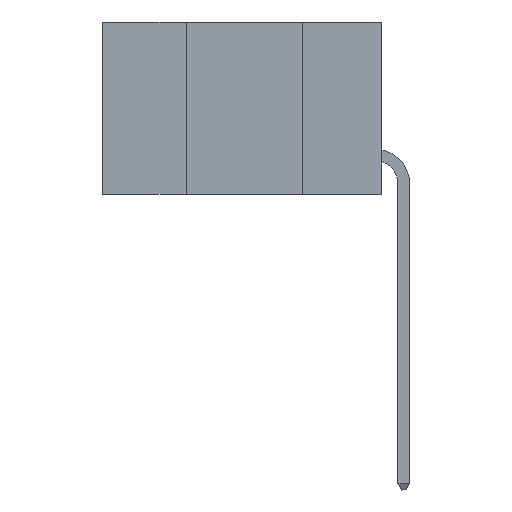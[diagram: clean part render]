
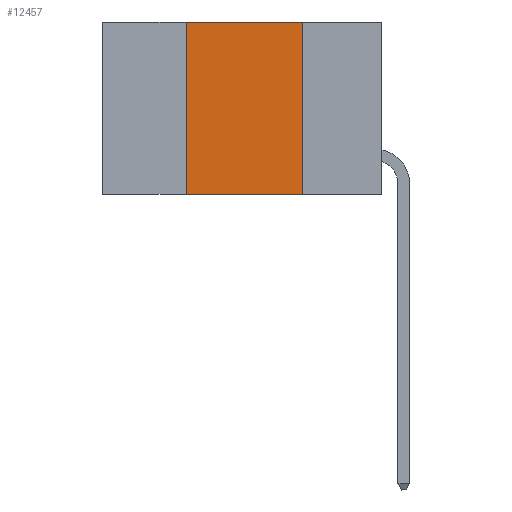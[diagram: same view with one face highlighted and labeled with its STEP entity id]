
A CAD part, left-side view. The second image highlights one B-rep face of the part: STEP entity #12457.
In plain terms, the highlighted planar face has unit normal (-1, 0, 0).
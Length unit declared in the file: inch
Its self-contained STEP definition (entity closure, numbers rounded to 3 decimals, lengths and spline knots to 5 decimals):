
#441 = FACE_OUTER_BOUND ( 'NONE', #1649, .T. ) ;
#693 = ORIENTED_EDGE ( 'NONE', *, *, #11333, .F. ) ;
#1159 = CARTESIAN_POINT ( 'NONE',  ( 0., 0.17, -0.37 ) ) ;
#1432 = PLANE ( 'NONE',  #2350 ) ;
#1484 = VECTOR ( 'NONE', #4089, 39.37008 ) ;
#1649 = EDGE_LOOP ( 'NONE', ( #8991, #9758, #693, #6693 ) ) ;
#2350 = AXIS2_PLACEMENT_3D ( 'NONE', #4327, #8266, #9296 ) ;
#3684 = CARTESIAN_POINT ( 'NONE',  ( 0., 0.42, 0. ) ) ;
#4001 = VECTOR ( 'NONE', #6410, 39.37008 ) ;
#4035 = DIRECTION ( 'NONE',  ( 0., 0., -1. ) ) ;
#4072 = CARTESIAN_POINT ( 'NONE',  ( 0., 0.17, 0. ) ) ;
#4089 = DIRECTION ( 'NONE',  ( 0., -1., 0. ) ) ;
#4327 = CARTESIAN_POINT ( 'NONE',  ( 0., 0.6, 0. ) ) ;
#5220 = EDGE_CURVE ( 'NONE', #11867, #8327, #10793, .T. ) ;
#5570 = CARTESIAN_POINT ( 'NONE',  ( 0., 0.42, -0.37 ) ) ;
#5764 = DIRECTION ( 'NONE',  ( 0., -1., 0. ) ) ;
#5848 = EDGE_CURVE ( 'NONE', #8327, #7571, #12030, .T. ) ;
#6033 = LINE ( 'NONE', #10726, #6475 ) ;
#6410 = DIRECTION ( 'NONE',  ( 0., 0., 1. ) ) ;
#6475 = VECTOR ( 'NONE', #5764, 39.37008 ) ;
#6693 = ORIENTED_EDGE ( 'NONE', *, *, #9318, .T. ) ;
#6971 = CARTESIAN_POINT ( 'NONE',  ( 0., 0.6, 0. ) ) ;
#6995 = VECTOR ( 'NONE', #4035, 39.37008 ) ;
#7571 = VERTEX_POINT ( 'NONE', #1159 ) ;
#8244 = LINE ( 'NONE', #9320, #4001 ) ;
#8266 = DIRECTION ( 'NONE',  ( 1., 0., 0. ) ) ;
#8327 = VERTEX_POINT ( 'NONE', #11159 ) ;
#8966 = VERTEX_POINT ( 'NONE', #5570 ) ;
#8991 = ORIENTED_EDGE ( 'NONE', *, *, #5848, .F. ) ;
#9296 = DIRECTION ( 'NONE',  ( 0., 0., -1. ) ) ;
#9318 = EDGE_CURVE ( 'NONE', #8966, #7571, #6033, .T. ) ;
#9320 = CARTESIAN_POINT ( 'NONE',  ( 0., 0.42, 0. ) ) ;
#9758 = ORIENTED_EDGE ( 'NONE', *, *, #5220, .F. ) ;
#10726 = CARTESIAN_POINT ( 'NONE',  ( 0., 0.6, -0.37 ) ) ;
#10793 = LINE ( 'NONE', #6971, #1484 ) ;
#11159 = CARTESIAN_POINT ( 'NONE',  ( 0., 0.17, 0. ) ) ;
#11333 = EDGE_CURVE ( 'NONE', #8966, #11867, #8244, .T. ) ;
#11867 = VERTEX_POINT ( 'NONE', #3684 ) ;
#12030 = LINE ( 'NONE', #4072, #6995 ) ;
#12457 = ADVANCED_FACE ( 'NONE', ( #441 ), #1432, .F. ) ;
